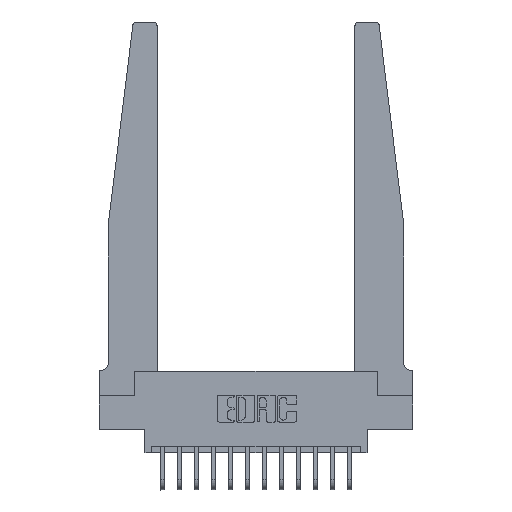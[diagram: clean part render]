
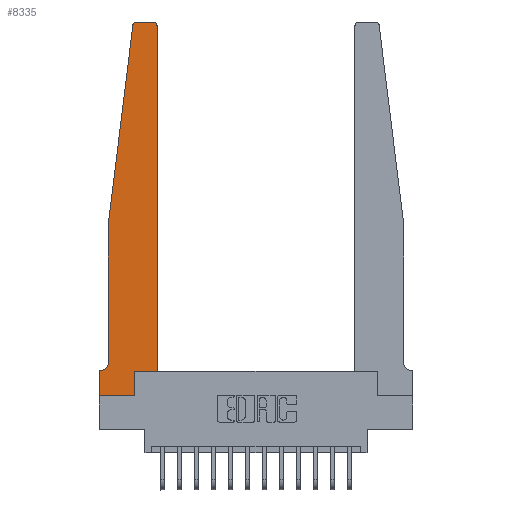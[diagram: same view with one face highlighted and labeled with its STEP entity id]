
A CAD part, top view. The second image highlights one B-rep face of the part: STEP entity #8335.
In plain terms, the highlighted planar face has unit normal (0, 0, 1).
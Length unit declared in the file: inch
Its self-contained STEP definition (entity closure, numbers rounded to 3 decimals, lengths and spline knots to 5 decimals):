
#591 = EDGE_CURVE ( 'NONE', #14444, #14906, #3004, .T. ) ;
#971 = VERTEX_POINT ( 'NONE', #12537 ) ;
#975 = VECTOR ( 'NONE', #12685, 39.37008 ) ;
#1138 = DIRECTION ( 'NONE',  ( 0., 0., 1. ) ) ;
#1331 = VECTOR ( 'NONE', #1861, 39.37008 ) ;
#1674 = VERTEX_POINT ( 'NONE', #10580 ) ;
#1748 = DIRECTION ( 'NONE',  ( -1., 0., 0. ) ) ;
#1861 = DIRECTION ( 'NONE',  ( 1., 0., 0. ) ) ;
#1898 = EDGE_CURVE ( 'NONE', #14906, #9579, #9667, .T. ) ;
#1903 = DIRECTION ( 'NONE',  ( 1., 0., 0. ) ) ;
#1945 = ORIENTED_EDGE ( 'NONE', *, *, #1898, .T. ) ;
#2354 = VERTEX_POINT ( 'NONE', #3093 ) ;
#2376 = DIRECTION ( 'NONE',  ( 1., 0., 0. ) ) ;
#2596 = EDGE_CURVE ( 'NONE', #1674, #2354, #10368, .T. ) ;
#2881 = VERTEX_POINT ( 'NONE', #16829 ) ;
#3004 = LINE ( 'NONE', #14770, #6632 ) ;
#3093 = CARTESIAN_POINT ( 'NONE',  ( 0.065, 0.2375, 0.37 ) ) ;
#3119 = CARTESIAN_POINT ( 'NONE',  ( 0.425, 2.72, 0.37 ) ) ;
#4154 = ORIENTED_EDGE ( 'NONE', *, *, #4339, .T. ) ;
#4231 = AXIS2_PLACEMENT_3D ( 'NONE', #5453, #1138, #2376 ) ;
#4339 = EDGE_CURVE ( 'NONE', #971, #14444, #17945, .T. ) ;
#4653 = CARTESIAN_POINT ( 'NONE',  ( 0., 0.1875, 0.37 ) ) ;
#4728 = ORIENTED_EDGE ( 'NONE', *, *, #5889, .T. ) ;
#4806 = EDGE_CURVE ( 'NONE', #10122, #7778, #7746, .T. ) ;
#4921 = DIRECTION ( 'NONE',  ( 1., 0., 0. ) ) ;
#5019 = ORIENTED_EDGE ( 'NONE', *, *, #2596, .T. ) ;
#5055 = EDGE_CURVE ( 'NONE', #2354, #10122, #18383, .T. ) ;
#5127 = CIRCLE ( 'NONE', #4231, 0.03 ) ;
#5390 = CARTESIAN_POINT ( 'NONE',  ( 0.25, 2.75, 0.37 ) ) ;
#5453 = CARTESIAN_POINT ( 'NONE',  ( 0.395, 2.72, 0.37 ) ) ;
#5747 = CIRCLE ( 'NONE', #11627, 0.03 ) ;
#5889 = EDGE_CURVE ( 'NONE', #9579, #5967, #6327, .T. ) ;
#5967 = VERTEX_POINT ( 'NONE', #3119 ) ;
#6327 = LINE ( 'NONE', #10879, #975 ) ;
#6422 = ORIENTED_EDGE ( 'NONE', *, *, #12009, .T. ) ;
#6423 = CARTESIAN_POINT ( 'NONE',  ( 0.015, 0.2375, 0.37 ) ) ;
#6586 = LINE ( 'NONE', #8312, #6944 ) ;
#6632 = VECTOR ( 'NONE', #7432, 39.37008 ) ;
#6720 = DIRECTION ( 'NONE',  ( 1., 0., 0. ) ) ;
#6848 = CARTESIAN_POINT ( 'NONE',  ( 0.2605, 0., 0.37 ) ) ;
#6926 = LINE ( 'NONE', #5390, #16497 ) ;
#6944 = VECTOR ( 'NONE', #9493, 39.37008 ) ;
#7280 = EDGE_CURVE ( 'NONE', #7778, #971, #6586, .T. ) ;
#7310 = VECTOR ( 'NONE', #13127, 39.37008 ) ;
#7432 = DIRECTION ( 'NONE',  ( 0., 1., 0. ) ) ;
#7579 = CARTESIAN_POINT ( 'NONE',  ( 0.24675, 2.72367, 0.37 ) ) ;
#7746 = LINE ( 'NONE', #9300, #15058 ) ;
#7778 = VERTEX_POINT ( 'NONE', #4653 ) ;
#8110 = EDGE_CURVE ( 'NONE', #18650, #2881, #6926, .T. ) ;
#8312 = CARTESIAN_POINT ( 'NONE',  ( 0., 0., 0.37 ) ) ;
#8335 = ADVANCED_FACE ( 'NONE', ( #13389 ), #16386, .T. ) ;
#8440 = EDGE_CURVE ( 'NONE', #2881, #15529, #5747, .T. ) ;
#8576 = EDGE_CURVE ( 'NONE', #5967, #18650, #5127, .T. ) ;
#9064 = ORIENTED_EDGE ( 'NONE', *, *, #8576, .T. ) ;
#9300 = CARTESIAN_POINT ( 'NONE',  ( 0.065, 0.1875, 0.37 ) ) ;
#9404 = CARTESIAN_POINT ( 'NONE',  ( 0.425, 0.18, 0.37 ) ) ;
#9493 = DIRECTION ( 'NONE',  ( 0., -1., 0. ) ) ;
#9579 = VERTEX_POINT ( 'NONE', #9404 ) ;
#9635 = CARTESIAN_POINT ( 'NONE',  ( 0.27653, 2.72, 0.37 ) ) ;
#9667 = LINE ( 'NONE', #18089, #16840 ) ;
#9974 = DIRECTION ( 'NONE',  ( -1., 0., 0. ) ) ;
#10053 = ORIENTED_EDGE ( 'NONE', *, *, #8440, .T. ) ;
#10122 = VERTEX_POINT ( 'NONE', #14538 ) ;
#10218 = VECTOR ( 'NONE', #18043, 39.37008 ) ;
#10368 = LINE ( 'NONE', #13216, #7310 ) ;
#10518 = CARTESIAN_POINT ( 'NONE',  ( 0.2605, 0.18, 0.37 ) ) ;
#10580 = CARTESIAN_POINT ( 'NONE',  ( 0.065, 1.25, 0.37 ) ) ;
#10879 = CARTESIAN_POINT ( 'NONE',  ( 0.425, 0.18, 0.37 ) ) ;
#10895 = DIRECTION ( 'NONE',  ( -1., 0., 0. ) ) ;
#11627 = AXIS2_PLACEMENT_3D ( 'NONE', #9635, #15393, #6720 ) ;
#12009 = EDGE_CURVE ( 'NONE', #15529, #1674, #16522, .T. ) ;
#12166 = CARTESIAN_POINT ( 'NONE',  ( 0., 0.1875, 0.37 ) ) ;
#12537 = CARTESIAN_POINT ( 'NONE',  ( 0., 0., 0.37 ) ) ;
#12685 = DIRECTION ( 'NONE',  ( 0., 1., 0. ) ) ;
#12748 = ORIENTED_EDGE ( 'NONE', *, *, #8110, .T. ) ;
#13127 = DIRECTION ( 'NONE',  ( 0., -1., 0. ) ) ;
#13216 = CARTESIAN_POINT ( 'NONE',  ( 0.065, 1.25, 0.37 ) ) ;
#13389 = FACE_OUTER_BOUND ( 'NONE', #17508, .T. ) ;
#14444 = VERTEX_POINT ( 'NONE', #6848 ) ;
#14538 = CARTESIAN_POINT ( 'NONE',  ( 0.015, 0.1875, 0.37 ) ) ;
#14770 = CARTESIAN_POINT ( 'NONE',  ( 0.2605, 0.18, 0.37 ) ) ;
#14906 = VERTEX_POINT ( 'NONE', #10518 ) ;
#15031 = AXIS2_PLACEMENT_3D ( 'NONE', #6423, #18149, #10895 ) ;
#15058 = VECTOR ( 'NONE', #1748, 39.37008 ) ;
#15381 = ORIENTED_EDGE ( 'NONE', *, *, #5055, .T. ) ;
#15393 = DIRECTION ( 'NONE',  ( 0., 0., 1. ) ) ;
#15529 = VERTEX_POINT ( 'NONE', #7579 ) ;
#15904 = AXIS2_PLACEMENT_3D ( 'NONE', #12166, #16472, #1903 ) ;
#16265 = ORIENTED_EDGE ( 'NONE', *, *, #7280, .T. ) ;
#16386 = PLANE ( 'NONE',  #15904 ) ;
#16472 = DIRECTION ( 'NONE',  ( 0., 0., 1. ) ) ;
#16497 = VECTOR ( 'NONE', #9974, 39.37008 ) ;
#16509 = CARTESIAN_POINT ( 'NONE',  ( 0., 0., 0.37 ) ) ;
#16522 = LINE ( 'NONE', #16622, #10218 ) ;
#16622 = CARTESIAN_POINT ( 'NONE',  ( 0.065, 1.25, 0.37 ) ) ;
#16625 = ORIENTED_EDGE ( 'NONE', *, *, #4806, .T. ) ;
#16829 = CARTESIAN_POINT ( 'NONE',  ( 0.27653, 2.75, 0.37 ) ) ;
#16840 = VECTOR ( 'NONE', #4921, 39.37008 ) ;
#17300 = ORIENTED_EDGE ( 'NONE', *, *, #591, .T. ) ;
#17508 = EDGE_LOOP ( 'NONE', ( #12748, #10053, #6422, #5019, #15381, #16625, #16265, #4154, #17300, #1945, #4728, #9064 ) ) ;
#17836 = CARTESIAN_POINT ( 'NONE',  ( 0.395, 2.75, 0.37 ) ) ;
#17945 = LINE ( 'NONE', #16509, #1331 ) ;
#18043 = DIRECTION ( 'NONE',  ( -0.122, -0.992, 0. ) ) ;
#18089 = CARTESIAN_POINT ( 'NONE',  ( 0.425, 0.18, 0.37 ) ) ;
#18149 = DIRECTION ( 'NONE',  ( 0., 0., -1. ) ) ;
#18383 = CIRCLE ( 'NONE', #15031, 0.05 ) ;
#18650 = VERTEX_POINT ( 'NONE', #17836 ) ;
